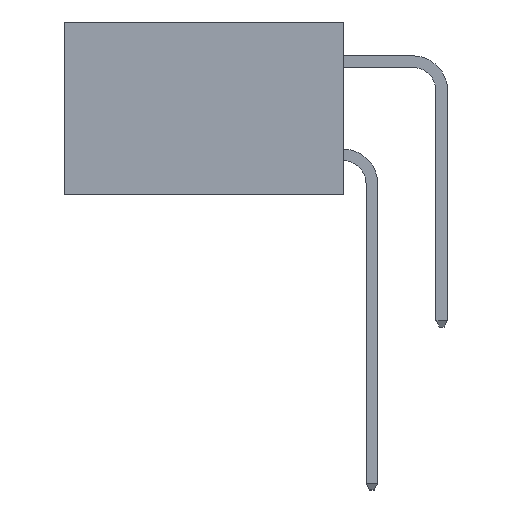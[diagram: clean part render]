
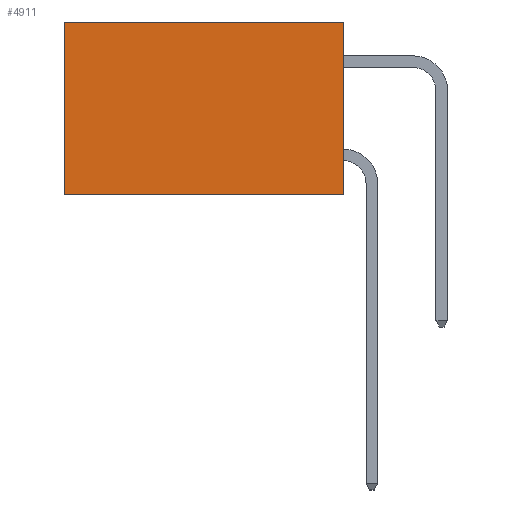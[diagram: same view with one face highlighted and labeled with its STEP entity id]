
A CAD part, left-side view. The second image highlights one B-rep face of the part: STEP entity #4911.
In plain terms, the highlighted planar face has unit normal (-1, 0, 0).
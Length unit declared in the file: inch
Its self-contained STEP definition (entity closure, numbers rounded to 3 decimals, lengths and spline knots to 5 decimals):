
#688 = CARTESIAN_POINT ( 'NONE',  ( 0.2615, 0.6, -0.37 ) ) ;
#955 = CARTESIAN_POINT ( 'NONE',  ( 0.2615, 0., 0. ) ) ;
#1056 = ORIENTED_EDGE ( 'NONE', *, *, #5806, .F. ) ;
#1145 = VECTOR ( 'NONE', #1981, 39.37008 ) ;
#1561 = VERTEX_POINT ( 'NONE', #688 ) ;
#1981 = DIRECTION ( 'NONE',  ( 0., 1., 0. ) ) ;
#2016 = CARTESIAN_POINT ( 'NONE',  ( 0.2615, 0., -0.37 ) ) ;
#2355 = CARTESIAN_POINT ( 'NONE',  ( 0.2615, 0., -0.37 ) ) ;
#2725 = LINE ( 'NONE', #2355, #8808 ) ;
#3235 = EDGE_LOOP ( 'NONE', ( #8329, #9969, #1056, #10239 ) ) ;
#3242 = DIRECTION ( 'NONE',  ( 0., 0., -1. ) ) ;
#3294 = LINE ( 'NONE', #6661, #9269 ) ;
#3812 = LINE ( 'NONE', #955, #1145 ) ;
#4081 = DIRECTION ( 'NONE',  ( 0., 0., -1. ) ) ;
#4180 = LINE ( 'NONE', #9951, #9769 ) ;
#4801 = CARTESIAN_POINT ( 'NONE',  ( 0.2615, 0., 0. ) ) ;
#4911 = ADVANCED_FACE ( 'NONE', ( #8270 ), #5726, .F. ) ;
#4982 = EDGE_CURVE ( 'NONE', #6837, #1561, #3294, .T. ) ;
#5427 = AXIS2_PLACEMENT_3D ( 'NONE', #6510, #8711, #4081 ) ;
#5494 = VERTEX_POINT ( 'NONE', #4801 ) ;
#5726 = PLANE ( 'NONE',  #5427 ) ;
#5806 = EDGE_CURVE ( 'NONE', #5494, #6837, #2725, .T. ) ;
#5900 = DIRECTION ( 'NONE',  ( 0., 1., 0. ) ) ;
#6331 = DIRECTION ( 'NONE',  ( 0., 0., -1. ) ) ;
#6510 = CARTESIAN_POINT ( 'NONE',  ( 0.2615, 0., -0.37 ) ) ;
#6661 = CARTESIAN_POINT ( 'NONE',  ( 0.2615, 0., -0.37 ) ) ;
#6770 = EDGE_CURVE ( 'NONE', #5494, #10440, #3812, .T. ) ;
#6837 = VERTEX_POINT ( 'NONE', #2016 ) ;
#7057 = CARTESIAN_POINT ( 'NONE',  ( 0.2615, 0.6, 0. ) ) ;
#8270 = FACE_OUTER_BOUND ( 'NONE', #3235, .T. ) ;
#8329 = ORIENTED_EDGE ( 'NONE', *, *, #10485, .T. ) ;
#8711 = DIRECTION ( 'NONE',  ( 1., 0., 0. ) ) ;
#8808 = VECTOR ( 'NONE', #3242, 39.37008 ) ;
#9269 = VECTOR ( 'NONE', #5900, 39.37008 ) ;
#9769 = VECTOR ( 'NONE', #6331, 39.37008 ) ;
#9951 = CARTESIAN_POINT ( 'NONE',  ( 0.2615, 0.6, -0.37 ) ) ;
#9969 = ORIENTED_EDGE ( 'NONE', *, *, #4982, .F. ) ;
#10239 = ORIENTED_EDGE ( 'NONE', *, *, #6770, .T. ) ;
#10440 = VERTEX_POINT ( 'NONE', #7057 ) ;
#10485 = EDGE_CURVE ( 'NONE', #10440, #1561, #4180, .T. ) ;
